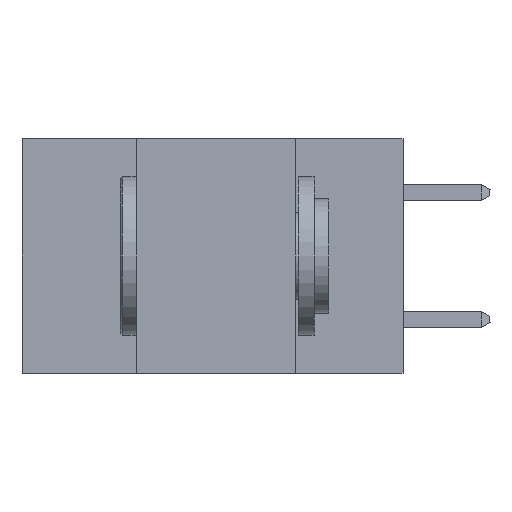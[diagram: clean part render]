
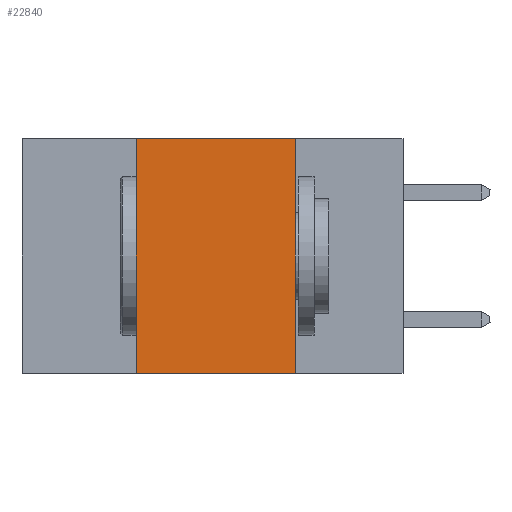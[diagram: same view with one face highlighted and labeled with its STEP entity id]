
A CAD part, left-side view. The second image highlights one B-rep face of the part: STEP entity #22840.
In plain terms, the highlighted planar face has unit normal (-1, 0, 0).
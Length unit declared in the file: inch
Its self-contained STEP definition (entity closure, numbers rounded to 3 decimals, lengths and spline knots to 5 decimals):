
#671 = CARTESIAN_POINT ( 'NONE',  ( 0., 0.17, 0. ) ) ;
#1732 = VERTEX_POINT ( 'NONE', #22707 ) ;
#2879 = DIRECTION ( 'NONE',  ( 0., -1., 0. ) ) ;
#3307 = LINE ( 'NONE', #3931, #32320 ) ;
#3931 = CARTESIAN_POINT ( 'NONE',  ( 0., 0.42, 0. ) ) ;
#4212 = ORIENTED_EDGE ( 'NONE', *, *, #15807, .F. ) ;
#5141 = LINE ( 'NONE', #671, #33223 ) ;
#5212 = DIRECTION ( 'NONE',  ( 0., -1., 0. ) ) ;
#5507 = ORIENTED_EDGE ( 'NONE', *, *, #25130, .F. ) ;
#7335 = EDGE_CURVE ( 'NONE', #1732, #8126, #3307, .T. ) ;
#7371 = VECTOR ( 'NONE', #5212, 39.37008 ) ;
#7828 = DIRECTION ( 'NONE',  ( 1., 0., 0. ) ) ;
#7888 = ORIENTED_EDGE ( 'NONE', *, *, #33295, .T. ) ;
#8126 = VERTEX_POINT ( 'NONE', #32366 ) ;
#8628 = CARTESIAN_POINT ( 'NONE',  ( 0., 0.6, 0. ) ) ;
#11394 = VECTOR ( 'NONE', #2879, 39.37008 ) ;
#12258 = VERTEX_POINT ( 'NONE', #17327 ) ;
#13379 = FACE_OUTER_BOUND ( 'NONE', #25315, .T. ) ;
#15407 = DIRECTION ( 'NONE',  ( 0., 0., 1. ) ) ;
#15807 = EDGE_CURVE ( 'NONE', #8126, #12258, #18014, .T. ) ;
#17327 = CARTESIAN_POINT ( 'NONE',  ( 0., 0.17, 0. ) ) ;
#17760 = DIRECTION ( 'NONE',  ( 0., 0., -1. ) ) ;
#18014 = LINE ( 'NONE', #8628, #11394 ) ;
#22137 = CARTESIAN_POINT ( 'NONE',  ( 0., 0.6, -0.37 ) ) ;
#22707 = CARTESIAN_POINT ( 'NONE',  ( 0., 0.42, -0.37 ) ) ;
#22840 = ADVANCED_FACE ( 'NONE', ( #13379 ), #32946, .F. ) ;
#24734 = CARTESIAN_POINT ( 'NONE',  ( 0., 0.6, 0. ) ) ;
#24923 = CARTESIAN_POINT ( 'NONE',  ( 0., 0.17, -0.37 ) ) ;
#25130 = EDGE_CURVE ( 'NONE', #12258, #33978, #5141, .T. ) ;
#25315 = EDGE_LOOP ( 'NONE', ( #5507, #4212, #29466, #7888 ) ) ;
#27559 = DIRECTION ( 'NONE',  ( 0., 0., -1. ) ) ;
#29466 = ORIENTED_EDGE ( 'NONE', *, *, #7335, .F. ) ;
#30657 = LINE ( 'NONE', #22137, #7371 ) ;
#32320 = VECTOR ( 'NONE', #15407, 39.37008 ) ;
#32366 = CARTESIAN_POINT ( 'NONE',  ( 0., 0.42, 0. ) ) ;
#32771 = AXIS2_PLACEMENT_3D ( 'NONE', #24734, #7828, #27559 ) ;
#32946 = PLANE ( 'NONE',  #32771 ) ;
#33223 = VECTOR ( 'NONE', #17760, 39.37008 ) ;
#33295 = EDGE_CURVE ( 'NONE', #1732, #33978, #30657, .T. ) ;
#33978 = VERTEX_POINT ( 'NONE', #24923 ) ;
